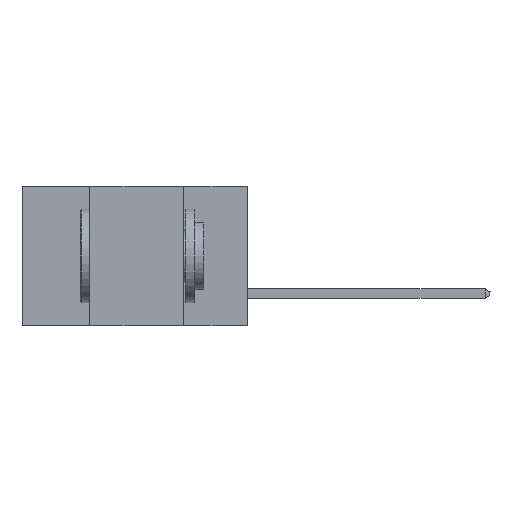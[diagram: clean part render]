
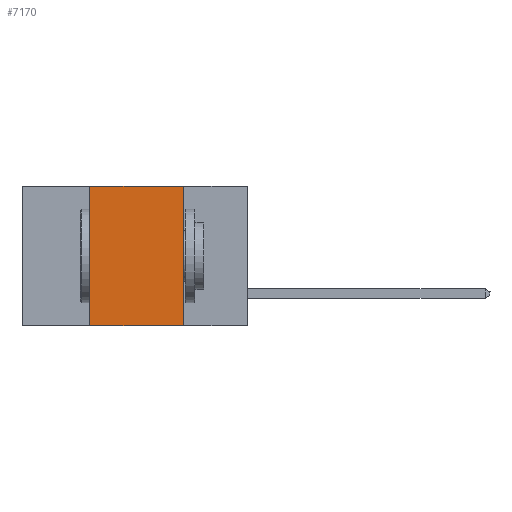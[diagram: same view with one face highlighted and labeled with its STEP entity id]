
A CAD part, left-side view. The second image highlights one B-rep face of the part: STEP entity #7170.
In plain terms, the highlighted planar face has unit normal (-1, 0, 0).
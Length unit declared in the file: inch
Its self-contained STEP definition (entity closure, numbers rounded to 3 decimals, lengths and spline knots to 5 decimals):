
#226 = ORIENTED_EDGE ( 'NONE', *, *, #2504, .T. ) ;
#760 = VERTEX_POINT ( 'NONE', #4775 ) ;
#1018 = DIRECTION ( 'NONE',  ( 0., -1., 0. ) ) ;
#1084 = CARTESIAN_POINT ( 'NONE',  ( 0., 0.6, -0.37 ) ) ;
#1179 = LINE ( 'NONE', #3154, #5764 ) ;
#1357 = VECTOR ( 'NONE', #1018, 39.37008 ) ;
#1456 = ORIENTED_EDGE ( 'NONE', *, *, #9875, .F. ) ;
#1522 = LINE ( 'NONE', #7874, #7783 ) ;
#1662 = EDGE_LOOP ( 'NONE', ( #12910, #1456, #2515, #226 ) ) ;
#1778 = PLANE ( 'NONE',  #6578 ) ;
#2072 = VERTEX_POINT ( 'NONE', #3214 ) ;
#2504 = EDGE_CURVE ( 'NONE', #5826, #5670, #3421, .T. ) ;
#2515 = ORIENTED_EDGE ( 'NONE', *, *, #12394, .F. ) ;
#3154 = CARTESIAN_POINT ( 'NONE',  ( 0., 0.17, -0.37 ) ) ;
#3214 = CARTESIAN_POINT ( 'NONE',  ( 0., 0.42, 0. ) ) ;
#3360 = DIRECTION ( 'NONE',  ( 0., 0., -1. ) ) ;
#3421 = LINE ( 'NONE', #1084, #1357 ) ;
#3767 = CARTESIAN_POINT ( 'NONE',  ( 0., 0.6, 0. ) ) ;
#4159 = DIRECTION ( 'NONE',  ( 0., -1., 0. ) ) ;
#4775 = CARTESIAN_POINT ( 'NONE',  ( 0., 0.17, 0. ) ) ;
#5127 = CARTESIAN_POINT ( 'NONE',  ( 0., 0.6, 0. ) ) ;
#5670 = VERTEX_POINT ( 'NONE', #12497 ) ;
#5764 = VECTOR ( 'NONE', #3360, 39.37008 ) ;
#5826 = VERTEX_POINT ( 'NONE', #10838 ) ;
#6162 = FACE_OUTER_BOUND ( 'NONE', #1662, .T. ) ;
#6578 = AXIS2_PLACEMENT_3D ( 'NONE', #3767, #12096, #6933 ) ;
#6933 = DIRECTION ( 'NONE',  ( 0., 0., -1. ) ) ;
#7170 = ADVANCED_FACE ( 'NONE', ( #6162 ), #1778, .F. ) ;
#7783 = VECTOR ( 'NONE', #9845, 39.37008 ) ;
#7874 = CARTESIAN_POINT ( 'NONE',  ( 0., 0.42, -0.37 ) ) ;
#9082 = EDGE_CURVE ( 'NONE', #760, #5670, #1179, .T. ) ;
#9845 = DIRECTION ( 'NONE',  ( 0., 0., 1. ) ) ;
#9875 = EDGE_CURVE ( 'NONE', #2072, #760, #12467, .T. ) ;
#10112 = VECTOR ( 'NONE', #4159, 39.37008 ) ;
#10838 = CARTESIAN_POINT ( 'NONE',  ( 0., 0.42, -0.37 ) ) ;
#12096 = DIRECTION ( 'NONE',  ( 1., 0., 0. ) ) ;
#12394 = EDGE_CURVE ( 'NONE', #5826, #2072, #1522, .T. ) ;
#12467 = LINE ( 'NONE', #5127, #10112 ) ;
#12497 = CARTESIAN_POINT ( 'NONE',  ( 0., 0.17, -0.37 ) ) ;
#12910 = ORIENTED_EDGE ( 'NONE', *, *, #9082, .F. ) ;
